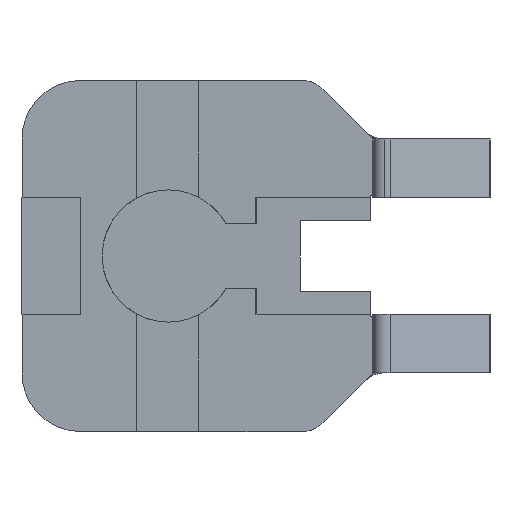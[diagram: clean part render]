
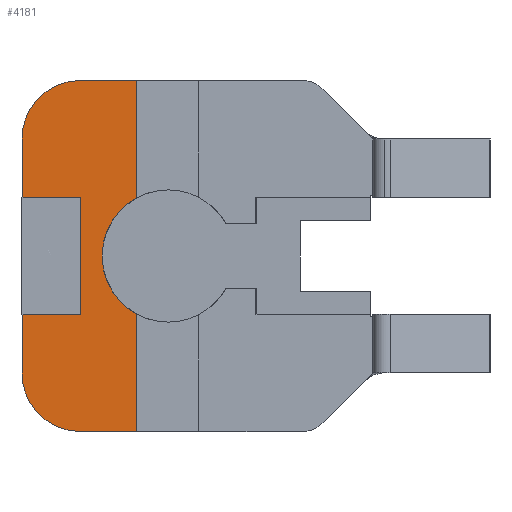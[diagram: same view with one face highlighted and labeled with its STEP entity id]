
A CAD part, left-side view. The second image highlights one B-rep face of the part: STEP entity #4181.
In plain terms, the highlighted planar face has unit normal (-1, 0, 0).
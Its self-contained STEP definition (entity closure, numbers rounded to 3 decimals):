
#19 = DIRECTION ( 'NONE',  ( 0., -1., 0. ) ) ;
#37 = VECTOR ( 'NONE', #1403, 1000. ) ;
#43 = VECTOR ( 'NONE', #2216, 1000. ) ;
#69 = AXIS2_PLACEMENT_3D ( 'NONE', #1918, #4278, #2263 ) ;
#142 = AXIS2_PLACEMENT_3D ( 'NONE', #1050, #3442, #1393 ) ;
#446 = VECTOR ( 'NONE', #1022, 1000. ) ;
#459 = CARTESIAN_POINT ( 'NONE',  ( 2.735, 30.792, -20. ) ) ;
#520 = LINE ( 'NONE', #2300, #4150 ) ;
#525 = VECTOR ( 'NONE', #1805, 1000. ) ;
#549 = VERTEX_POINT ( 'NONE', #1177 ) ;
#599 = AXIS2_PLACEMENT_3D ( 'NONE', #3735, #1680, #4063 ) ;
#629 = EDGE_LOOP ( 'NONE', ( #2640, #2840, #2023, #2759, #4071, #3737, #1953, #4182, #1119, #1960, #3799, #2719 ) ) ;
#631 = LINE ( 'NONE', #1456, #525 ) ;
#759 = CARTESIAN_POINT ( 'NONE',  ( 2.735, 35.792, 0. ) ) ;
#867 = FACE_OUTER_BOUND ( 'NONE', #629, .T. ) ;
#890 = VERTEX_POINT ( 'NONE', #1573 ) ;
#924 = VERTEX_POINT ( 'NONE', #4001 ) ;
#939 = LINE ( 'NONE', #2531, #43 ) ;
#947 = CARTESIAN_POINT ( 'NONE',  ( 2.735, 35.792, 5. ) ) ;
#1022 = DIRECTION ( 'NONE',  ( 0., 1., 0. ) ) ;
#1050 = CARTESIAN_POINT ( 'NONE',  ( 2.735, 23.292, -5. ) ) ;
#1067 = EDGE_CURVE ( 'NONE', #890, #3417, #2486, .T. ) ;
#1119 = ORIENTED_EDGE ( 'NONE', *, *, #1155, .F. ) ;
#1128 = EDGE_CURVE ( 'NONE', #549, #1571, #2277, .T. ) ;
#1129 = VECTOR ( 'NONE', #3846, 1000. ) ;
#1155 = EDGE_CURVE ( 'NONE', #3417, #2787, #2974, .T. ) ;
#1177 = CARTESIAN_POINT ( 'NONE',  ( 2.735, 30.792, 0. ) ) ;
#1209 = EDGE_CURVE ( 'NONE', #1571, #890, #1852, .T. ) ;
#1236 = EDGE_CURVE ( 'NONE', #2787, #924, #2645, .T. ) ;
#1272 = DIRECTION ( 'NONE',  ( 0., 0., -1. ) ) ;
#1374 = CARTESIAN_POINT ( 'NONE',  ( 2.735, 25.992, 10. ) ) ;
#1393 = DIRECTION ( 'NONE',  ( 0., 0., -1. ) ) ;
#1403 = DIRECTION ( 'NONE',  ( 0., 0., 1. ) ) ;
#1416 = EDGE_CURVE ( 'NONE', #4136, #3310, #939, .T. ) ;
#1456 = CARTESIAN_POINT ( 'NONE',  ( 2.735, 30.792, -10. ) ) ;
#1496 = CARTESIAN_POINT ( 'NONE',  ( 2.735, 30.792, -10. ) ) ;
#1505 = EDGE_CURVE ( 'NONE', #3310, #3964, #4132, .T. ) ;
#1554 = CARTESIAN_POINT ( 'NONE',  ( 2.735, 30.792, 10. ) ) ;
#1566 = DIRECTION ( 'NONE',  ( 1., 0., 0. ) ) ;
#1571 = VERTEX_POINT ( 'NONE', #759 ) ;
#1573 = CARTESIAN_POINT ( 'NONE',  ( 2.735, 35.792, 5. ) ) ;
#1606 = VECTOR ( 'NONE', #3017, 1000. ) ;
#1680 = DIRECTION ( 'NONE',  ( 1., 0., 0. ) ) ;
#1721 = CARTESIAN_POINT ( 'NONE',  ( 2.735, 30.792, 10. ) ) ;
#1804 = CARTESIAN_POINT ( 'NONE',  ( 2.735, 35.792, -10. ) ) ;
#1805 = DIRECTION ( 'NONE',  ( 0., 0., 1. ) ) ;
#1831 = EDGE_CURVE ( 'NONE', #3964, #4036, #2525, .T. ) ;
#1852 = LINE ( 'NONE', #2097, #37 ) ;
#1918 = CARTESIAN_POINT ( 'NONE',  ( 2.735, 11.828, 7.5 ) ) ;
#1953 = ORIENTED_EDGE ( 'NONE', *, *, #1974, .T. ) ;
#1960 = ORIENTED_EDGE ( 'NONE', *, *, #1067, .F. ) ;
#1974 = EDGE_CURVE ( 'NONE', #2659, #924, #3907, .T. ) ;
#2023 = ORIENTED_EDGE ( 'NONE', *, *, #1831, .F. ) ;
#2097 = CARTESIAN_POINT ( 'NONE',  ( 2.735, 35.792, 5. ) ) ;
#2148 = EDGE_CURVE ( 'NONE', #4036, #3334, #3852, .T. ) ;
#2162 = CARTESIAN_POINT ( 'NONE',  ( 2.735, 25.992, -20. ) ) ;
#2216 = DIRECTION ( 'NONE',  ( 0., 1., 0. ) ) ;
#2263 = DIRECTION ( 'NONE',  ( 0., 0., 1. ) ) ;
#2277 = LINE ( 'NONE', #3751, #446 ) ;
#2300 = CARTESIAN_POINT ( 'NONE',  ( 2.735, 25.992, 20. ) ) ;
#2335 = CARTESIAN_POINT ( 'NONE',  ( 2.735, 25.992, -9.963 ) ) ;
#2365 = AXIS2_PLACEMENT_3D ( 'NONE', #3624, #1566, #4350 ) ;
#2448 = EDGE_CURVE ( 'NONE', #3334, #549, #631, .T. ) ;
#2486 = CIRCLE ( 'NONE', #599, 5. ) ;
#2525 = LINE ( 'NONE', #947, #1606 ) ;
#2531 = CARTESIAN_POINT ( 'NONE',  ( 2.735, 11.828, -20. ) ) ;
#2640 = ORIENTED_EDGE ( 'NONE', *, *, #2448, .F. ) ;
#2645 = LINE ( 'NONE', #2795, #4288 ) ;
#2659 = VERTEX_POINT ( 'NONE', #2335 ) ;
#2719 = ORIENTED_EDGE ( 'NONE', *, *, #1128, .F. ) ;
#2759 = ORIENTED_EDGE ( 'NONE', *, *, #1505, .F. ) ;
#2787 = VERTEX_POINT ( 'NONE', #1374 ) ;
#2795 = CARTESIAN_POINT ( 'NONE',  ( 2.735, 25.992, 20. ) ) ;
#2840 = ORIENTED_EDGE ( 'NONE', *, *, #2148, .F. ) ;
#2866 = VECTOR ( 'NONE', #19, 1000. ) ;
#2901 = EDGE_CURVE ( 'NONE', #2659, #4136, #520, .T. ) ;
#2974 = LINE ( 'NONE', #1721, #2866 ) ;
#3017 = DIRECTION ( 'NONE',  ( 0., 0., 1. ) ) ;
#3310 = VERTEX_POINT ( 'NONE', #459 ) ;
#3334 = VERTEX_POINT ( 'NONE', #1496 ) ;
#3417 = VERTEX_POINT ( 'NONE', #1554 ) ;
#3442 = DIRECTION ( 'NONE',  ( 1., 0., 0. ) ) ;
#3624 = CARTESIAN_POINT ( 'NONE',  ( 2.735, 30.792, -15. ) ) ;
#3735 = CARTESIAN_POINT ( 'NONE',  ( 2.735, 30.792, 5. ) ) ;
#3737 = ORIENTED_EDGE ( 'NONE', *, *, #2901, .F. ) ;
#3751 = CARTESIAN_POINT ( 'NONE',  ( 2.735, 35.792, 0. ) ) ;
#3799 = ORIENTED_EDGE ( 'NONE', *, *, #1209, .F. ) ;
#3803 = CARTESIAN_POINT ( 'NONE',  ( 2.735, 35.792, -15. ) ) ;
#3811 = DIRECTION ( 'NONE',  ( 0., 0., -1. ) ) ;
#3846 = DIRECTION ( 'NONE',  ( 0., -1., 0. ) ) ;
#3852 = LINE ( 'NONE', #1804, #1129 ) ;
#3907 = CIRCLE ( 'NONE', #142, 5.65 ) ;
#3952 = PLANE ( 'NONE',  #69 ) ;
#3964 = VERTEX_POINT ( 'NONE', #3803 ) ;
#4001 = CARTESIAN_POINT ( 'NONE',  ( 2.735, 25.992, -0.037 ) ) ;
#4036 = VERTEX_POINT ( 'NONE', #4153 ) ;
#4063 = DIRECTION ( 'NONE',  ( 0., 0., -1. ) ) ;
#4071 = ORIENTED_EDGE ( 'NONE', *, *, #1416, .F. ) ;
#4132 = CIRCLE ( 'NONE', #2365, 5. ) ;
#4136 = VERTEX_POINT ( 'NONE', #2162 ) ;
#4150 = VECTOR ( 'NONE', #1272, 1000. ) ;
#4153 = CARTESIAN_POINT ( 'NONE',  ( 2.735, 35.792, -10. ) ) ;
#4181 = ADVANCED_FACE ( 'NONE', ( #867 ), #3952, .T. ) ;
#4182 = ORIENTED_EDGE ( 'NONE', *, *, #1236, .F. ) ;
#4278 = DIRECTION ( 'NONE',  ( -1., 0., 0. ) ) ;
#4288 = VECTOR ( 'NONE', #3811, 1000. ) ;
#4350 = DIRECTION ( 'NONE',  ( 0., 0., 1. ) ) ;
